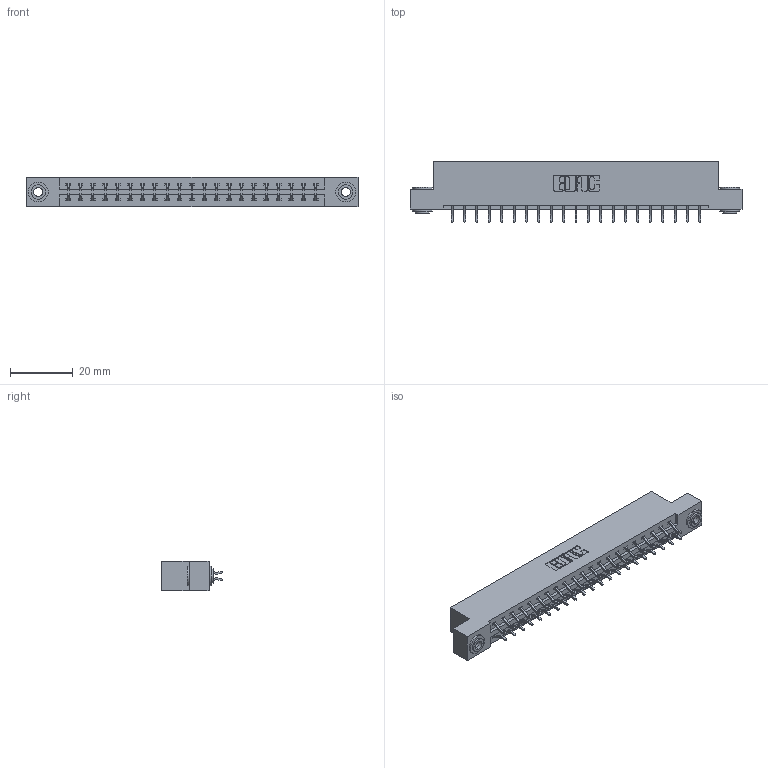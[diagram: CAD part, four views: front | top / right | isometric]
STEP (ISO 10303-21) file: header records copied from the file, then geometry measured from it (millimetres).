
FILE_DESCRIPTION (( 'STEP AP203' ), '1' );
FILE_NAME ('387-042-556-203.STEP', '2018-09-19T23:26:16', ( '' ), ( '' ), 'SwSTEP 2.0', 'SolidWorks 2016', '' );
FILE_SCHEMA (( 'CONFIG_CONTROL_DESIGN' ));
Length unit declared in the file: inch
Products named in the file (4): 337 Part_Flush Mounting Lugs - 0.156 Dia-TH; 345-292-001_556 Tail; 345-250-002_345-250-002-102; 387-042-556-203
Assembly tree (45 placements, depth 2):
  387-042-556-203
    337 Part_Flush Mounting Lugs - 0.156 Dia-TH
    345-292-001_556 Tail  x42
    345-250-002_345-250-002-102  x2
Bounding box: 106.22 x 19.57 x 9.4 mm (x, y, z)
Volume: 10932.8 mm3; surface area: 12335.7 mm2
Topology: 45 solids, 45 shells, 2672 faces, 7905 edges, 5210 vertices
Faces by surface type: plane 1844, cylinder 820, cone 8
Entity records: 19868 total; most frequent: CARTESIAN_POINT 3353, ORIENTED_EDGE 3270, DIRECTION 2913, EDGE_CURVE 1635, LINE 1475, VECTOR 1475, VERTEX_POINT 1086, AXIS2_PLACEMENT_3D 719
